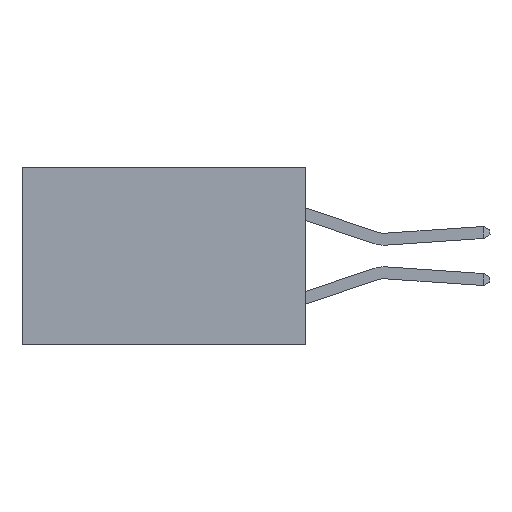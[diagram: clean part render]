
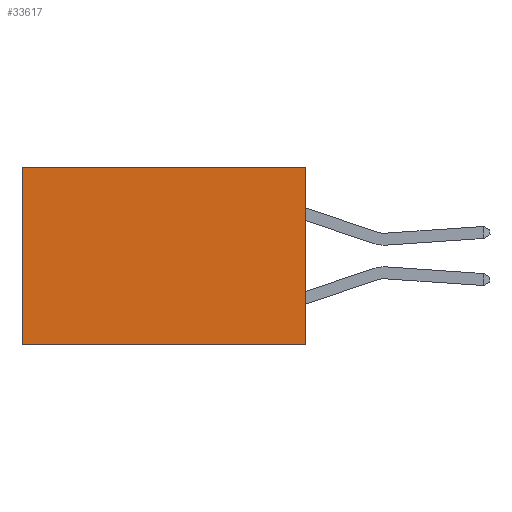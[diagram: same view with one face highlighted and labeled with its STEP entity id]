
A CAD part, left-side view. The second image highlights one B-rep face of the part: STEP entity #33617.
In plain terms, the highlighted planar face has unit normal (-1, 0, 0).
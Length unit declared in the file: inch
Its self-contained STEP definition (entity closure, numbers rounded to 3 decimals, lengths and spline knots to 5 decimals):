
#1992 = LINE ( 'NONE', #18003, #15263 ) ;
#2170 = DIRECTION ( 'NONE',  ( 0., 1., 0. ) ) ;
#2291 = CARTESIAN_POINT ( 'NONE',  ( 0.277, 0., -0.37 ) ) ;
#2785 = VECTOR ( 'NONE', #17814, 39.37008 ) ;
#3374 = AXIS2_PLACEMENT_3D ( 'NONE', #2291, #5023, #23384 ) ;
#3584 = CARTESIAN_POINT ( 'NONE',  ( 0.277, 0., 0. ) ) ;
#4664 = EDGE_LOOP ( 'NONE', ( #18660, #30429, #31392, #9308 ) ) ;
#5023 = DIRECTION ( 'NONE',  ( 1., 0., 0. ) ) ;
#6789 = CARTESIAN_POINT ( 'NONE',  ( 0.277, 0.59, -0.37 ) ) ;
#7636 = VERTEX_POINT ( 'NONE', #10201 ) ;
#9232 = CARTESIAN_POINT ( 'NONE',  ( 0.277, 0., 0. ) ) ;
#9308 = ORIENTED_EDGE ( 'NONE', *, *, #13679, .T. ) ;
#9833 = LINE ( 'NONE', #22979, #2785 ) ;
#10201 = CARTESIAN_POINT ( 'NONE',  ( 0.277, 0., -0.37 ) ) ;
#11923 = DIRECTION ( 'NONE',  ( 0., 1., 0. ) ) ;
#12557 = LINE ( 'NONE', #6789, #25665 ) ;
#12839 = LINE ( 'NONE', #9232, #32758 ) ;
#13679 = EDGE_CURVE ( 'NONE', #14331, #13683, #12839, .T. ) ;
#13683 = VERTEX_POINT ( 'NONE', #32698 ) ;
#14331 = VERTEX_POINT ( 'NONE', #3584 ) ;
#14914 = CARTESIAN_POINT ( 'NONE',  ( 0.277, 0.59, -0.37 ) ) ;
#15263 = VECTOR ( 'NONE', #2170, 39.37008 ) ;
#17814 = DIRECTION ( 'NONE',  ( 0., 0., -1. ) ) ;
#18003 = CARTESIAN_POINT ( 'NONE',  ( 0.277, 0., -0.37 ) ) ;
#18113 = PLANE ( 'NONE',  #3374 ) ;
#18660 = ORIENTED_EDGE ( 'NONE', *, *, #19621, .T. ) ;
#19621 = EDGE_CURVE ( 'NONE', #13683, #30206, #12557, .T. ) ;
#21268 = EDGE_CURVE ( 'NONE', #7636, #30206, #1992, .T. ) ;
#22979 = CARTESIAN_POINT ( 'NONE',  ( 0.277, 0., -0.37 ) ) ;
#23384 = DIRECTION ( 'NONE',  ( 0., 0., -1. ) ) ;
#25665 = VECTOR ( 'NONE', #27764, 39.37008 ) ;
#27764 = DIRECTION ( 'NONE',  ( 0., 0., -1. ) ) ;
#27803 = EDGE_CURVE ( 'NONE', #14331, #7636, #9833, .T. ) ;
#30206 = VERTEX_POINT ( 'NONE', #14914 ) ;
#30429 = ORIENTED_EDGE ( 'NONE', *, *, #21268, .F. ) ;
#31392 = ORIENTED_EDGE ( 'NONE', *, *, #27803, .F. ) ;
#31419 = FACE_OUTER_BOUND ( 'NONE', #4664, .T. ) ;
#32698 = CARTESIAN_POINT ( 'NONE',  ( 0.277, 0.59, 0. ) ) ;
#32758 = VECTOR ( 'NONE', #11923, 39.37008 ) ;
#33617 = ADVANCED_FACE ( 'NONE', ( #31419 ), #18113, .F. ) ;
